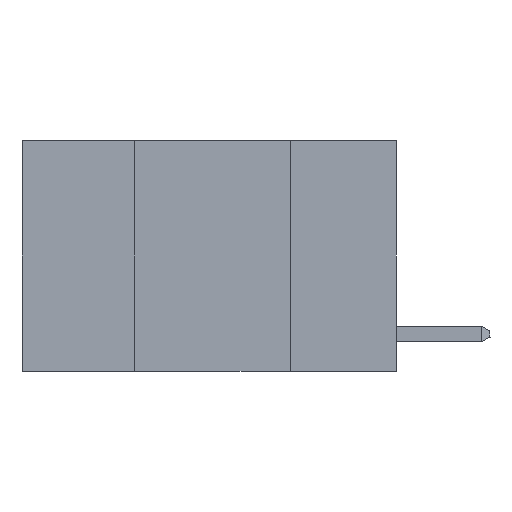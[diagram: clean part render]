
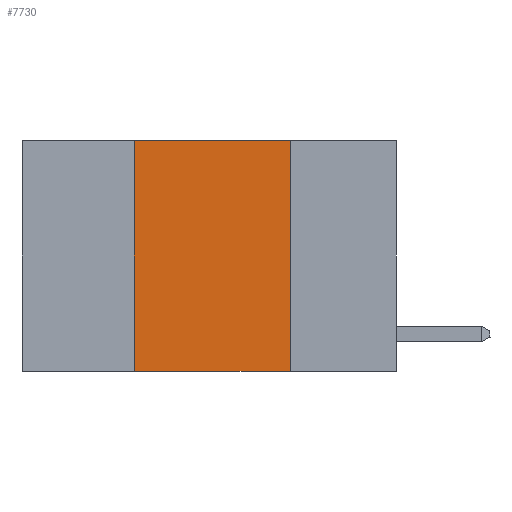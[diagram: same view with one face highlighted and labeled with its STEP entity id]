
A CAD part, left-side view. The second image highlights one B-rep face of the part: STEP entity #7730.
In plain terms, the highlighted planar face has unit normal (-1, 0, 0).
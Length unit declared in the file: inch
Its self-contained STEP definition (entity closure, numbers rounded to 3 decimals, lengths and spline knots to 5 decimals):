
#81 = VECTOR ( 'NONE', #1725, 39.37008 ) ;
#205 = CARTESIAN_POINT ( 'NONE',  ( 0., 0.6, 0. ) ) ;
#480 = EDGE_LOOP ( 'NONE', ( #7760, #9272, #2732, #4547 ) ) ;
#1250 = DIRECTION ( 'NONE',  ( 0., 0., -1. ) ) ;
#1725 = DIRECTION ( 'NONE',  ( 0., 0., -1. ) ) ;
#1834 = CARTESIAN_POINT ( 'NONE',  ( 0., 0.17, 0. ) ) ;
#2325 = VERTEX_POINT ( 'NONE', #8903 ) ;
#2694 = VERTEX_POINT ( 'NONE', #6414 ) ;
#2732 = ORIENTED_EDGE ( 'NONE', *, *, #9605, .F. ) ;
#2906 = LINE ( 'NONE', #1834, #81 ) ;
#2959 = EDGE_CURVE ( 'NONE', #6470, #2325, #4386, .T. ) ;
#3313 = EDGE_CURVE ( 'NONE', #2325, #5938, #2906, .T. ) ;
#3950 = AXIS2_PLACEMENT_3D ( 'NONE', #205, #7525, #1250 ) ;
#4069 = VECTOR ( 'NONE', #4332, 39.37008 ) ;
#4332 = DIRECTION ( 'NONE',  ( 0., -1., 0. ) ) ;
#4346 = CARTESIAN_POINT ( 'NONE',  ( 0., 0.6, 0. ) ) ;
#4386 = LINE ( 'NONE', #4346, #4069 ) ;
#4547 = ORIENTED_EDGE ( 'NONE', *, *, #10490, .T. ) ;
#4812 = VECTOR ( 'NONE', #6476, 39.37008 ) ;
#5457 = CARTESIAN_POINT ( 'NONE',  ( 0., 0.6, -0.37 ) ) ;
#5938 = VERTEX_POINT ( 'NONE', #12734 ) ;
#6146 = VECTOR ( 'NONE', #6936, 39.37008 ) ;
#6414 = CARTESIAN_POINT ( 'NONE',  ( 0., 0.42, -0.37 ) ) ;
#6470 = VERTEX_POINT ( 'NONE', #12520 ) ;
#6476 = DIRECTION ( 'NONE',  ( 0., -1., 0. ) ) ;
#6936 = DIRECTION ( 'NONE',  ( 0., 0., 1. ) ) ;
#7525 = DIRECTION ( 'NONE',  ( 1., 0., 0. ) ) ;
#7730 = ADVANCED_FACE ( 'NONE', ( #10148 ), #11450, .F. ) ;
#7760 = ORIENTED_EDGE ( 'NONE', *, *, #3313, .F. ) ;
#8850 = LINE ( 'NONE', #8961, #6146 ) ;
#8903 = CARTESIAN_POINT ( 'NONE',  ( 0., 0.17, 0. ) ) ;
#8961 = CARTESIAN_POINT ( 'NONE',  ( 0., 0.42, 0. ) ) ;
#9272 = ORIENTED_EDGE ( 'NONE', *, *, #2959, .F. ) ;
#9605 = EDGE_CURVE ( 'NONE', #2694, #6470, #8850, .T. ) ;
#10148 = FACE_OUTER_BOUND ( 'NONE', #480, .T. ) ;
#10490 = EDGE_CURVE ( 'NONE', #2694, #5938, #12447, .T. ) ;
#11450 = PLANE ( 'NONE',  #3950 ) ;
#12447 = LINE ( 'NONE', #5457, #4812 ) ;
#12520 = CARTESIAN_POINT ( 'NONE',  ( 0., 0.42, 0. ) ) ;
#12734 = CARTESIAN_POINT ( 'NONE',  ( 0., 0.17, -0.37 ) ) ;
